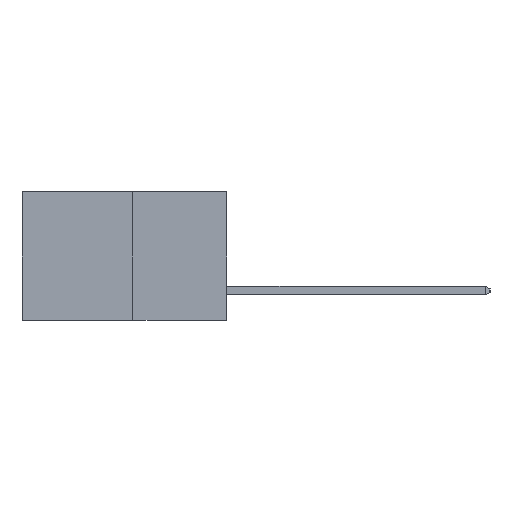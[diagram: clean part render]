
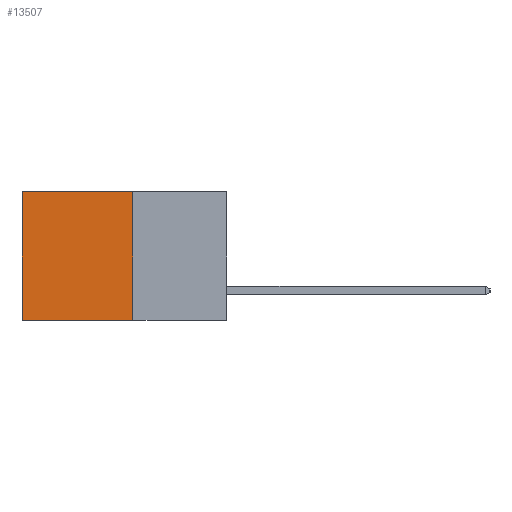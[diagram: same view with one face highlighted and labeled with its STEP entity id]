
A CAD part, left-side view. The second image highlights one B-rep face of the part: STEP entity #13507.
In plain terms, the highlighted planar face has unit normal (-1, 0, 0).
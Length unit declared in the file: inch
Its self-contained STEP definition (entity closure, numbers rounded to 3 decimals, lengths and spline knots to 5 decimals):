
#191 = CARTESIAN_POINT ( 'NONE',  ( 0.277, 0.59, -0.37 ) ) ;
#212 = DIRECTION ( 'NONE',  ( 0., 0., -1. ) ) ;
#721 = CARTESIAN_POINT ( 'NONE',  ( 0.277, 0.27, 0. ) ) ;
#774 = AXIS2_PLACEMENT_3D ( 'NONE', #4288, #11516, #5348 ) ;
#1519 = FACE_OUTER_BOUND ( 'NONE', #2216, .T. ) ;
#1733 = LINE ( 'NONE', #8117, #6683 ) ;
#1736 = CARTESIAN_POINT ( 'NONE',  ( 0.277, 0.27, 0. ) ) ;
#2183 = VECTOR ( 'NONE', #3518, 39.37008 ) ;
#2216 = EDGE_LOOP ( 'NONE', ( #2661, #4882, #6847, #9116 ) ) ;
#2661 = ORIENTED_EDGE ( 'NONE', *, *, #3962, .T. ) ;
#2924 = DIRECTION ( 'NONE',  ( 0., 1., 0. ) ) ;
#3518 = DIRECTION ( 'NONE',  ( 0., 0., -1. ) ) ;
#3962 = EDGE_CURVE ( 'NONE', #13335, #8461, #10148, .T. ) ;
#4288 = CARTESIAN_POINT ( 'NONE',  ( 0.277, 0.27, -0.37 ) ) ;
#4557 = CARTESIAN_POINT ( 'NONE',  ( 0.277, 0.27, -0.37 ) ) ;
#4882 = ORIENTED_EDGE ( 'NONE', *, *, #9067, .F. ) ;
#5251 = PLANE ( 'NONE',  #774 ) ;
#5348 = DIRECTION ( 'NONE',  ( 0., 0., -1. ) ) ;
#5972 = DIRECTION ( 'NONE',  ( 0., 1., 0. ) ) ;
#6087 = CARTESIAN_POINT ( 'NONE',  ( 0.277, 0.59, 0. ) ) ;
#6683 = VECTOR ( 'NONE', #2924, 39.37008 ) ;
#6847 = ORIENTED_EDGE ( 'NONE', *, *, #11798, .F. ) ;
#7062 = VECTOR ( 'NONE', #212, 39.37008 ) ;
#7706 = LINE ( 'NONE', #1736, #12803 ) ;
#7915 = CARTESIAN_POINT ( 'NONE',  ( 0.277, 0.27, -0.37 ) ) ;
#8032 = CARTESIAN_POINT ( 'NONE',  ( 0.277, 0.59, -0.37 ) ) ;
#8033 = VERTEX_POINT ( 'NONE', #721 ) ;
#8117 = CARTESIAN_POINT ( 'NONE',  ( 0.277, 0.27, -0.37 ) ) ;
#8461 = VERTEX_POINT ( 'NONE', #8032 ) ;
#9067 = EDGE_CURVE ( 'NONE', #11936, #8461, #1733, .T. ) ;
#9116 = ORIENTED_EDGE ( 'NONE', *, *, #12631, .T. ) ;
#10148 = LINE ( 'NONE', #191, #7062 ) ;
#11516 = DIRECTION ( 'NONE',  ( 1., 0., 0. ) ) ;
#11798 = EDGE_CURVE ( 'NONE', #8033, #11936, #13429, .T. ) ;
#11936 = VERTEX_POINT ( 'NONE', #7915 ) ;
#12631 = EDGE_CURVE ( 'NONE', #8033, #13335, #7706, .T. ) ;
#12803 = VECTOR ( 'NONE', #5972, 39.37008 ) ;
#13335 = VERTEX_POINT ( 'NONE', #6087 ) ;
#13429 = LINE ( 'NONE', #4557, #2183 ) ;
#13507 = ADVANCED_FACE ( 'NONE', ( #1519 ), #5251, .F. ) ;
